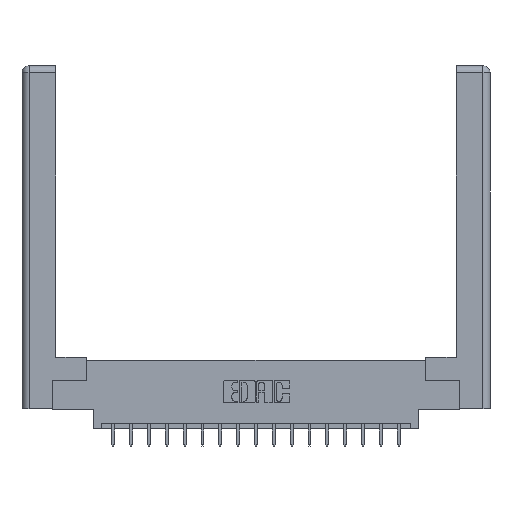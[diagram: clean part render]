
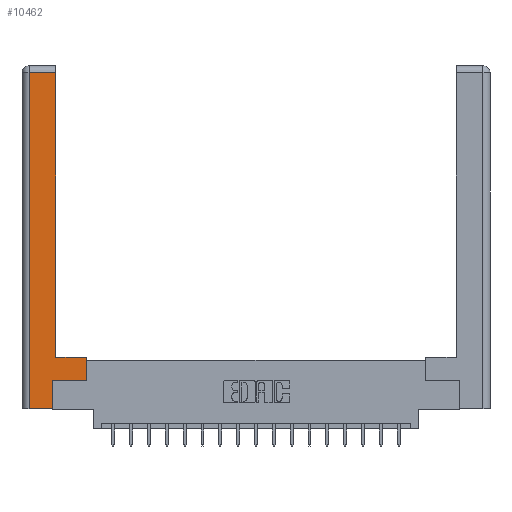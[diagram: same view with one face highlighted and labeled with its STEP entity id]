
A CAD part, top view. The second image highlights one B-rep face of the part: STEP entity #10462.
In plain terms, the highlighted planar face has unit normal (0, 0, 1).
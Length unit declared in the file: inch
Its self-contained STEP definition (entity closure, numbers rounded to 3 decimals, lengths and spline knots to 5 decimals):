
#1117 = ORIENTED_EDGE ( 'NONE', *, *, #13289, .T. ) ;
#1133 = EDGE_LOOP ( 'NONE', ( #15264, #4707, #2641, #12794, #1117, #6789, #5536, #10611 ) ) ;
#1261 = DIRECTION ( 'NONE',  ( -1., 0., 0. ) ) ;
#1355 = CARTESIAN_POINT ( 'NONE',  ( 0.265, 0.245, 0. ) ) ;
#2294 = CARTESIAN_POINT ( 'NONE',  ( 0.265, 0., 0. ) ) ;
#2641 = ORIENTED_EDGE ( 'NONE', *, *, #6100, .T. ) ;
#2685 = EDGE_CURVE ( 'NONE', #16471, #9229, #11321, .T. ) ;
#2875 = LINE ( 'NONE', #12846, #17487 ) ;
#3684 = CARTESIAN_POINT ( 'NONE',  ( 0.265, 0., 0. ) ) ;
#3812 = CARTESIAN_POINT ( 'NONE',  ( 0.565, 0.45, 0. ) ) ;
#3907 = CARTESIAN_POINT ( 'NONE',  ( 0.265, 0.245, 0. ) ) ;
#4707 = ORIENTED_EDGE ( 'NONE', *, *, #2685, .T. ) ;
#5536 = ORIENTED_EDGE ( 'NONE', *, *, #18249, .T. ) ;
#5670 = DIRECTION ( 'NONE',  ( 0., 1., 0. ) ) ;
#5770 = VECTOR ( 'NONE', #8176, 39.37008 ) ;
#6100 = EDGE_CURVE ( 'NONE', #9229, #16513, #17243, .T. ) ;
#6789 = ORIENTED_EDGE ( 'NONE', *, *, #13523, .T. ) ;
#6932 = CARTESIAN_POINT ( 'NONE',  ( 0.0615, 2.94, 0. ) ) ;
#8176 = DIRECTION ( 'NONE',  ( 0., 1., 0. ) ) ;
#8539 = VERTEX_POINT ( 'NONE', #17413 ) ;
#8567 = EDGE_CURVE ( 'NONE', #18942, #16471, #10623, .T. ) ;
#8597 = CARTESIAN_POINT ( 'NONE',  ( 0.295, 3., 0. ) ) ;
#8763 = CARTESIAN_POINT ( 'NONE',  ( 0.0615, 0., 0. ) ) ;
#9229 = VERTEX_POINT ( 'NONE', #12113 ) ;
#9650 = DIRECTION ( 'NONE',  ( 1., 0., 0. ) ) ;
#9657 = DIRECTION ( 'NONE',  ( -1., 0., 0. ) ) ;
#10121 = CARTESIAN_POINT ( 'NONE',  ( 0.295, 0.45, 0. ) ) ;
#10155 = DIRECTION ( 'NONE',  ( 0., 1., 0. ) ) ;
#10388 = CARTESIAN_POINT ( 'NONE',  ( 0.295, 2.94, 0. ) ) ;
#10462 = ADVANCED_FACE ( 'NONE', ( #13393 ), #14069, .F. ) ;
#10479 = VERTEX_POINT ( 'NONE', #3812 ) ;
#10611 = ORIENTED_EDGE ( 'NONE', *, *, #15326, .T. ) ;
#10623 = LINE ( 'NONE', #8597, #12936 ) ;
#11186 = AXIS2_PLACEMENT_3D ( 'NONE', #15478, #15546, #12618 ) ;
#11321 = LINE ( 'NONE', #6932, #14584 ) ;
#12113 = CARTESIAN_POINT ( 'NONE',  ( 0.0615, 2.94, 0. ) ) ;
#12518 = LINE ( 'NONE', #10121, #13219 ) ;
#12618 = DIRECTION ( 'NONE',  ( -1., 0., 0. ) ) ;
#12794 = ORIENTED_EDGE ( 'NONE', *, *, #18278, .T. ) ;
#12829 = VECTOR ( 'NONE', #10155, 39.37008 ) ;
#12846 = CARTESIAN_POINT ( 'NONE',  ( 0.565, 0.245, 0. ) ) ;
#12936 = VECTOR ( 'NONE', #5670, 39.37008 ) ;
#13219 = VECTOR ( 'NONE', #1261, 39.37008 ) ;
#13284 = VERTEX_POINT ( 'NONE', #1355 ) ;
#13289 = EDGE_CURVE ( 'NONE', #14052, #13284, #16798, .T. ) ;
#13393 = FACE_OUTER_BOUND ( 'NONE', #1133, .T. ) ;
#13523 = EDGE_CURVE ( 'NONE', #13284, #8539, #2875, .T. ) ;
#14052 = VERTEX_POINT ( 'NONE', #2294 ) ;
#14069 = PLANE ( 'NONE',  #11186 ) ;
#14211 = CARTESIAN_POINT ( 'NONE',  ( 0.565, 0.45, 0. ) ) ;
#14552 = LINE ( 'NONE', #3684, #15940 ) ;
#14584 = VECTOR ( 'NONE', #9657, 39.37008 ) ;
#15264 = ORIENTED_EDGE ( 'NONE', *, *, #8567, .T. ) ;
#15326 = EDGE_CURVE ( 'NONE', #10479, #18942, #12518, .T. ) ;
#15478 = CARTESIAN_POINT ( 'NONE',  ( 0., 0., 0. ) ) ;
#15493 = CARTESIAN_POINT ( 'NONE',  ( 0.0615, 0., 0. ) ) ;
#15546 = DIRECTION ( 'NONE',  ( 0., 0., -1. ) ) ;
#15940 = VECTOR ( 'NONE', #9650, 39.37008 ) ;
#16034 = CARTESIAN_POINT ( 'NONE',  ( 0.295, 0.45, 0. ) ) ;
#16471 = VERTEX_POINT ( 'NONE', #10388 ) ;
#16513 = VERTEX_POINT ( 'NONE', #8763 ) ;
#16798 = LINE ( 'NONE', #3907, #12829 ) ;
#17243 = LINE ( 'NONE', #15493, #18637 ) ;
#17413 = CARTESIAN_POINT ( 'NONE',  ( 0.565, 0.245, 0. ) ) ;
#17471 = DIRECTION ( 'NONE',  ( 1., 0., 0. ) ) ;
#17487 = VECTOR ( 'NONE', #17471, 39.37008 ) ;
#17826 = LINE ( 'NONE', #14211, #5770 ) ;
#18249 = EDGE_CURVE ( 'NONE', #8539, #10479, #17826, .T. ) ;
#18278 = EDGE_CURVE ( 'NONE', #16513, #14052, #14552, .T. ) ;
#18315 = DIRECTION ( 'NONE',  ( 0., -1., 0. ) ) ;
#18637 = VECTOR ( 'NONE', #18315, 39.37008 ) ;
#18942 = VERTEX_POINT ( 'NONE', #16034 ) ;
